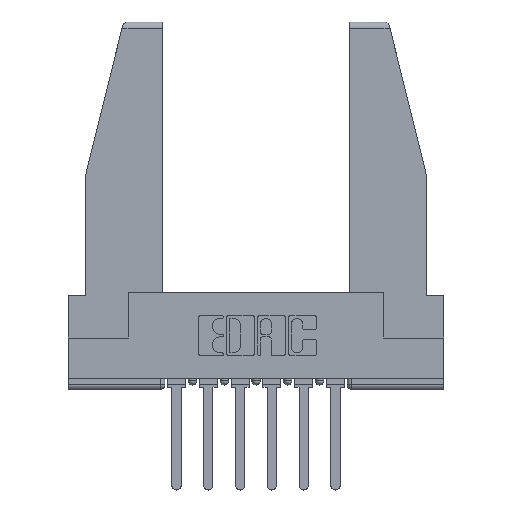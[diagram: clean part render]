
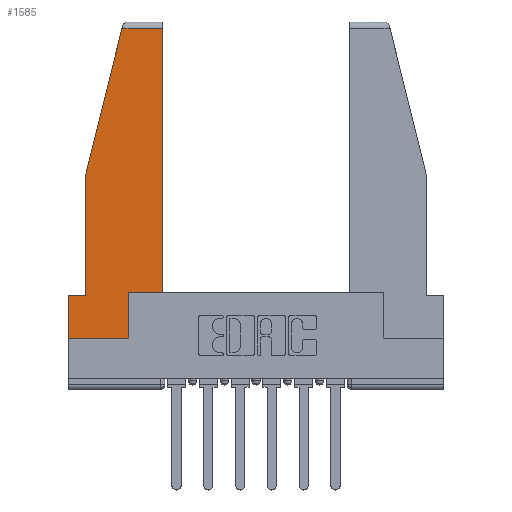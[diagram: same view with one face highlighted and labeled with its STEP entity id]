
A CAD part, top view. The second image highlights one B-rep face of the part: STEP entity #1585.
In plain terms, the highlighted planar face has unit normal (0, 0, 1).
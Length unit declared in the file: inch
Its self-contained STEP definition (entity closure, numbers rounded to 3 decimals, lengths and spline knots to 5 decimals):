
#13 = CARTESIAN_POINT ( 'NONE',  ( 0.086, 0.8, 0. ) ) ;
#247 = DIRECTION ( 'NONE',  ( 1., 0., 0. ) ) ;
#316 = VERTEX_POINT ( 'NONE', #3539 ) ;
#318 = VECTOR ( 'NONE', #3602, 39.37008 ) ;
#338 = EDGE_CURVE ( 'NONE', #316, #2117, #3675, .T. ) ;
#380 = CARTESIAN_POINT ( 'NONE',  ( 0.297, 0.223, 0. ) ) ;
#965 = CARTESIAN_POINT ( 'NONE',  ( 0.297, 0., 0. ) ) ;
#1474 = AXIS2_PLACEMENT_3D ( 'NONE', #2564, #7553, #8520 ) ;
#1585 = ADVANCED_FACE ( 'NONE', ( #8772 ), #3680, .T. ) ;
#1724 = CARTESIAN_POINT ( 'NONE',  ( 0.271, 1.55, 0. ) ) ;
#2117 = VERTEX_POINT ( 'NONE', #12621 ) ;
#2317 = CARTESIAN_POINT ( 'NONE',  ( 0.461, 0.223, 0. ) ) ;
#2564 = CARTESIAN_POINT ( 'NONE',  ( 0., 0., 0. ) ) ;
#2638 = ORIENTED_EDGE ( 'NONE', *, *, #12271, .T. ) ;
#3231 = LINE ( 'NONE', #13, #11717 ) ;
#3539 = CARTESIAN_POINT ( 'NONE',  ( 0.2636, 1.52, 0. ) ) ;
#3602 = DIRECTION ( 'NONE',  ( 1., 0., 0. ) ) ;
#3675 = LINE ( 'NONE', #1724, #7064 ) ;
#3680 = PLANE ( 'NONE',  #1474 ) ;
#3727 = LINE ( 'NONE', #4710, #318 ) ;
#3764 = CARTESIAN_POINT ( 'NONE',  ( 0.297, 0.223, 0. ) ) ;
#3922 = CARTESIAN_POINT ( 'NONE',  ( 0.297, 0., 0. ) ) ;
#3965 = VERTEX_POINT ( 'NONE', #3764 ) ;
#4009 = DIRECTION ( 'NONE',  ( 0., 1., 0. ) ) ;
#4174 = DIRECTION ( 'NONE',  ( -1., 0., 0. ) ) ;
#4710 = CARTESIAN_POINT ( 'NONE',  ( 0., 0., 0. ) ) ;
#4840 = VECTOR ( 'NONE', #4174, 39.37008 ) ;
#5219 = ORIENTED_EDGE ( 'NONE', *, *, #338, .T. ) ;
#5231 = ORIENTED_EDGE ( 'NONE', *, *, #5477, .T. ) ;
#5328 = ORIENTED_EDGE ( 'NONE', *, *, #5471, .T. ) ;
#5404 = CARTESIAN_POINT ( 'NONE',  ( 0., 0.21, 0. ) ) ;
#5471 = EDGE_CURVE ( 'NONE', #2117, #10609, #3231, .T. ) ;
#5477 = EDGE_CURVE ( 'NONE', #8945, #8104, #6013, .T. ) ;
#5543 = VECTOR ( 'NONE', #4009, 39.37008 ) ;
#5700 = VERTEX_POINT ( 'NONE', #8735 ) ;
#5998 = LINE ( 'NONE', #965, #6059 ) ;
#6013 = LINE ( 'NONE', #11046, #5543 ) ;
#6059 = VECTOR ( 'NONE', #7749, 39.37008 ) ;
#6200 = ORIENTED_EDGE ( 'NONE', *, *, #11760, .T. ) ;
#6282 = VERTEX_POINT ( 'NONE', #3922 ) ;
#6303 = DIRECTION ( 'NONE',  ( 0., -1., 0. ) ) ;
#6374 = CARTESIAN_POINT ( 'NONE',  ( 0., 0.21, 0. ) ) ;
#6409 = EDGE_CURVE ( 'NONE', #8104, #316, #10379, .T. ) ;
#6568 = LINE ( 'NONE', #12445, #8778 ) ;
#7064 = VECTOR ( 'NONE', #12582, 39.37008 ) ;
#7338 = CARTESIAN_POINT ( 'NONE',  ( 0., 1.52, 0. ) ) ;
#7553 = DIRECTION ( 'NONE',  ( 0., 0., 1. ) ) ;
#7749 = DIRECTION ( 'NONE',  ( 0., 1., 0. ) ) ;
#8104 = VERTEX_POINT ( 'NONE', #9153 ) ;
#8520 = DIRECTION ( 'NONE',  ( 1., 0., 0. ) ) ;
#8679 = ORIENTED_EDGE ( 'NONE', *, *, #9503, .T. ) ;
#8735 = CARTESIAN_POINT ( 'NONE',  ( 0., 0., 0. ) ) ;
#8772 = FACE_OUTER_BOUND ( 'NONE', #12657, .T. ) ;
#8778 = VECTOR ( 'NONE', #12312, 39.37008 ) ;
#8945 = VERTEX_POINT ( 'NONE', #2317 ) ;
#9153 = CARTESIAN_POINT ( 'NONE',  ( 0.461, 1.52, 0. ) ) ;
#9280 = ORIENTED_EDGE ( 'NONE', *, *, #12261, .T. ) ;
#9392 = VECTOR ( 'NONE', #6303, 39.37008 ) ;
#9503 = EDGE_CURVE ( 'NONE', #5700, #6282, #3727, .T. ) ;
#10127 = LINE ( 'NONE', #380, #10792 ) ;
#10144 = DIRECTION ( 'NONE',  ( 0., -1., 0. ) ) ;
#10206 = ORIENTED_EDGE ( 'NONE', *, *, #11587, .T. ) ;
#10379 = LINE ( 'NONE', #7338, #4840 ) ;
#10473 = ORIENTED_EDGE ( 'NONE', *, *, #6409, .T. ) ;
#10609 = VERTEX_POINT ( 'NONE', #11284 ) ;
#10792 = VECTOR ( 'NONE', #247, 39.37008 ) ;
#11023 = VERTEX_POINT ( 'NONE', #5404 ) ;
#11046 = CARTESIAN_POINT ( 'NONE',  ( 0.461, 0.223, 0. ) ) ;
#11284 = CARTESIAN_POINT ( 'NONE',  ( 0.086, 0.21, 0. ) ) ;
#11411 = LINE ( 'NONE', #6374, #9392 ) ;
#11587 = EDGE_CURVE ( 'NONE', #6282, #3965, #5998, .T. ) ;
#11717 = VECTOR ( 'NONE', #10144, 39.37008 ) ;
#11760 = EDGE_CURVE ( 'NONE', #3965, #8945, #10127, .T. ) ;
#12261 = EDGE_CURVE ( 'NONE', #11023, #5700, #11411, .T. ) ;
#12271 = EDGE_CURVE ( 'NONE', #10609, #11023, #6568, .T. ) ;
#12312 = DIRECTION ( 'NONE',  ( -1., 0., 0. ) ) ;
#12445 = CARTESIAN_POINT ( 'NONE',  ( 0., 0.21, 0. ) ) ;
#12582 = DIRECTION ( 'NONE',  ( -0.239, -0.971, 0. ) ) ;
#12621 = CARTESIAN_POINT ( 'NONE',  ( 0.086, 0.8, 0. ) ) ;
#12657 = EDGE_LOOP ( 'NONE', ( #5231, #10473, #5219, #5328, #2638, #9280, #8679, #10206, #6200 ) ) ;
